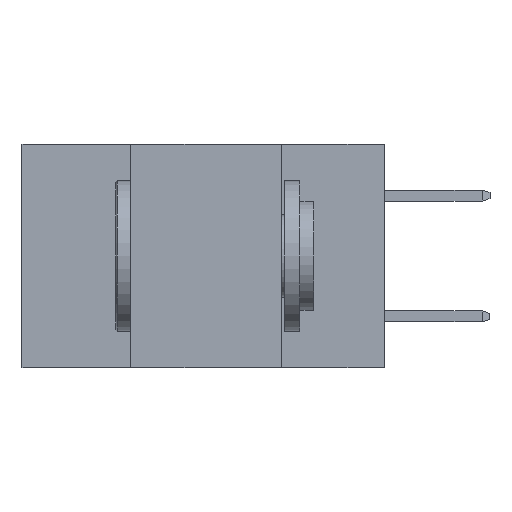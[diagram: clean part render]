
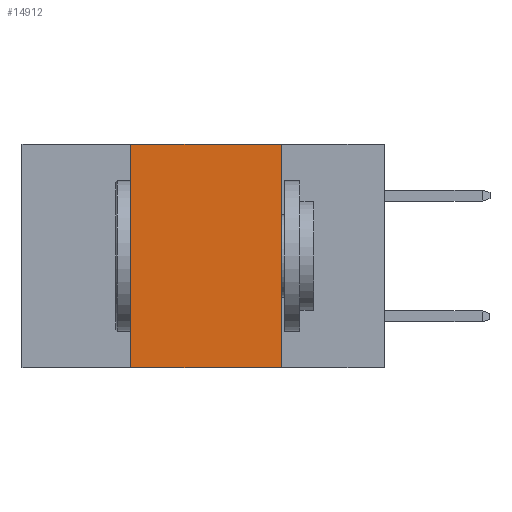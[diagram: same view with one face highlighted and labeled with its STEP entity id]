
A CAD part, left-side view. The second image highlights one B-rep face of the part: STEP entity #14912.
In plain terms, the highlighted planar face has unit normal (-1, 0, 0).
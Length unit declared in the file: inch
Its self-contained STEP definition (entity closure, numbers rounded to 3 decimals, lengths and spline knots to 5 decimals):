
#742 = LINE ( 'NONE', #3182, #14042 ) ;
#1089 = CARTESIAN_POINT ( 'NONE',  ( 0., 0.6, 0. ) ) ;
#1354 = VECTOR ( 'NONE', #24765, 39.37008 ) ;
#1400 = VERTEX_POINT ( 'NONE', #5615 ) ;
#3182 = CARTESIAN_POINT ( 'NONE',  ( 0., 0.6, -0.37 ) ) ;
#3618 = DIRECTION ( 'NONE',  ( 0., 0., -1. ) ) ;
#4137 = FACE_OUTER_BOUND ( 'NONE', #25415, .T. ) ;
#5615 = CARTESIAN_POINT ( 'NONE',  ( 0., 0.42, 0. ) ) ;
#7421 = VECTOR ( 'NONE', #9247, 39.37008 ) ;
#8184 = LINE ( 'NONE', #9040, #20676 ) ;
#8383 = VERTEX_POINT ( 'NONE', #28251 ) ;
#9040 = CARTESIAN_POINT ( 'NONE',  ( 0., 0.6, 0. ) ) ;
#9247 = DIRECTION ( 'NONE',  ( 0., 0., 1. ) ) ;
#11709 = CARTESIAN_POINT ( 'NONE',  ( 0., 0.42, -0.37 ) ) ;
#11989 = VERTEX_POINT ( 'NONE', #11709 ) ;
#12268 = ORIENTED_EDGE ( 'NONE', *, *, #23299, .F. ) ;
#12342 = CARTESIAN_POINT ( 'NONE',  ( 0., 0.17, -0.37 ) ) ;
#12403 = EDGE_CURVE ( 'NONE', #11989, #30180, #742, .T. ) ;
#14042 = VECTOR ( 'NONE', #20649, 39.37008 ) ;
#14063 = LINE ( 'NONE', #28999, #7421 ) ;
#14912 = ADVANCED_FACE ( 'NONE', ( #4137 ), #28407, .F. ) ;
#17255 = CARTESIAN_POINT ( 'NONE',  ( 0., 0.17, 0. ) ) ;
#18149 = AXIS2_PLACEMENT_3D ( 'NONE', #1089, #18568, #3618 ) ;
#18568 = DIRECTION ( 'NONE',  ( 1., 0., 0. ) ) ;
#19711 = ORIENTED_EDGE ( 'NONE', *, *, #29296, .F. ) ;
#20649 = DIRECTION ( 'NONE',  ( 0., -1., 0. ) ) ;
#20676 = VECTOR ( 'NONE', #26568, 39.37008 ) ;
#22901 = EDGE_CURVE ( 'NONE', #11989, #1400, #14063, .T. ) ;
#23299 = EDGE_CURVE ( 'NONE', #1400, #8383, #8184, .T. ) ;
#24765 = DIRECTION ( 'NONE',  ( 0., 0., -1. ) ) ;
#25415 = EDGE_LOOP ( 'NONE', ( #19711, #12268, #29596, #30110 ) ) ;
#26568 = DIRECTION ( 'NONE',  ( 0., -1., 0. ) ) ;
#27872 = LINE ( 'NONE', #17255, #1354 ) ;
#28251 = CARTESIAN_POINT ( 'NONE',  ( 0., 0.17, 0. ) ) ;
#28407 = PLANE ( 'NONE',  #18149 ) ;
#28999 = CARTESIAN_POINT ( 'NONE',  ( 0., 0.42, 0. ) ) ;
#29296 = EDGE_CURVE ( 'NONE', #8383, #30180, #27872, .T. ) ;
#29596 = ORIENTED_EDGE ( 'NONE', *, *, #22901, .F. ) ;
#30110 = ORIENTED_EDGE ( 'NONE', *, *, #12403, .T. ) ;
#30180 = VERTEX_POINT ( 'NONE', #12342 ) ;
